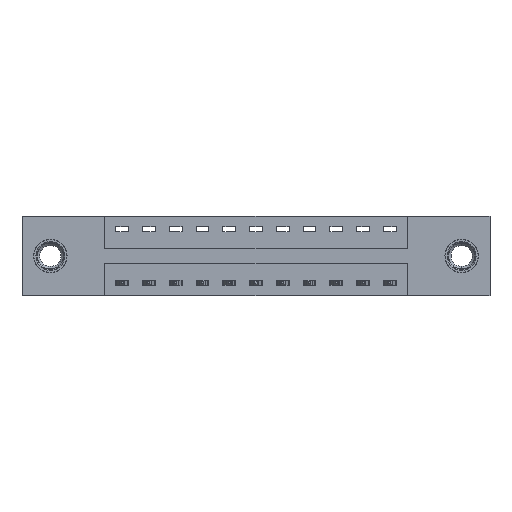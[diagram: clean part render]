
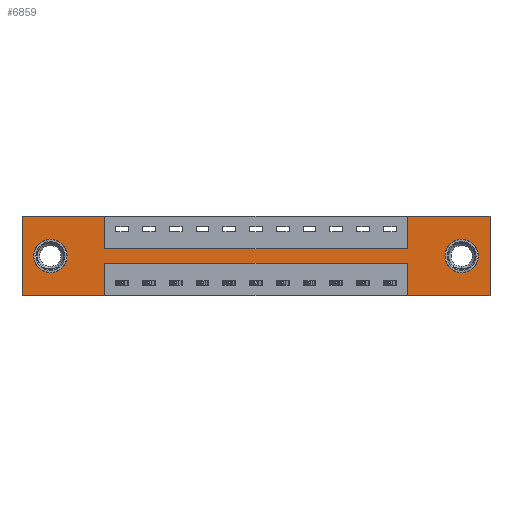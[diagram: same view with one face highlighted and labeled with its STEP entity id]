
A CAD part, front view. The second image highlights one B-rep face of the part: STEP entity #6859.
In plain terms, the highlighted planar face has unit normal (0, -1, 0).
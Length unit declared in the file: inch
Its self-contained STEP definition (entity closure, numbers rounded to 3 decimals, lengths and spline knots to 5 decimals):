
#109 = VERTEX_POINT ( 'NONE', #2069 ) ;
#162 = VERTEX_POINT ( 'NONE', #5123 ) ;
#343 = ORIENTED_EDGE ( 'NONE', *, *, #11135, .F. ) ;
#410 = CARTESIAN_POINT ( 'NONE',  ( 1.7975, 0., -0.15 ) ) ;
#486 = CARTESIAN_POINT ( 'NONE',  ( 1.7975, 0., -0.22 ) ) ;
#488 = EDGE_CURVE ( 'NONE', #7572, #2030, #11193, .T. ) ;
#491 = ORIENTED_EDGE ( 'NONE', *, *, #5879, .F. ) ;
#593 = VERTEX_POINT ( 'NONE', #3154 ) ;
#762 = CARTESIAN_POINT ( 'NONE',  ( 0.1325, 0., -0.185 ) ) ;
#849 = DIRECTION ( 'NONE',  ( 0., 0., 1. ) ) ;
#923 = CARTESIAN_POINT ( 'NONE',  ( 0., 0., 0. ) ) ;
#945 = LINE ( 'NONE', #8394, #10133 ) ;
#1381 = CARTESIAN_POINT ( 'NONE',  ( 0., 0., -0.37 ) ) ;
#1407 = CARTESIAN_POINT ( 'NONE',  ( 2.185, 0., 0. ) ) ;
#1415 = VECTOR ( 'NONE', #11627, 39.37008 ) ;
#1430 = ORIENTED_EDGE ( 'NONE', *, *, #6796, .F. ) ;
#1726 = LINE ( 'NONE', #923, #4914 ) ;
#1750 = DIRECTION ( 'NONE',  ( 0., -1., 0. ) ) ;
#1914 = VECTOR ( 'NONE', #849, 39.37008 ) ;
#1993 = FACE_OUTER_BOUND ( 'NONE', #2025, .T. ) ;
#2002 = LINE ( 'NONE', #5742, #10921 ) ;
#2025 = EDGE_LOOP ( 'NONE', ( #8663, #9573, #8241, #4562, #7363, #1430, #6151, #2543, #343, #491, #8839, #10587 ) ) ;
#2030 = VERTEX_POINT ( 'NONE', #11125 ) ;
#2040 = CARTESIAN_POINT ( 'NONE',  ( 2.0525, 0., -0.185 ) ) ;
#2069 = CARTESIAN_POINT ( 'NONE',  ( 0.3875, 0., 0. ) ) ;
#2076 = LINE ( 'NONE', #5697, #12197 ) ;
#2270 = DIRECTION ( 'NONE',  ( 0., 0., -1. ) ) ;
#2543 = ORIENTED_EDGE ( 'NONE', *, *, #9388, .F. ) ;
#2697 = DIRECTION ( 'NONE',  ( 0., 0., 1. ) ) ;
#2711 = DIRECTION ( 'NONE',  ( 0., 0., 1. ) ) ;
#2770 = CARTESIAN_POINT ( 'NONE',  ( 2.0525, 0., -0.107 ) ) ;
#2814 = ORIENTED_EDGE ( 'NONE', *, *, #6087, .T. ) ;
#2875 = VERTEX_POINT ( 'NONE', #1407 ) ;
#2902 = AXIS2_PLACEMENT_3D ( 'NONE', #3178, #3237, #8682 ) ;
#3089 = EDGE_CURVE ( 'NONE', #2030, #11890, #2076, .T. ) ;
#3128 = CARTESIAN_POINT ( 'NONE',  ( 2.0525, 0., -0.185 ) ) ;
#3154 = CARTESIAN_POINT ( 'NONE',  ( 1.7975, 0., 0. ) ) ;
#3178 = CARTESIAN_POINT ( 'NONE',  ( 0.1325, 0., -0.185 ) ) ;
#3237 = DIRECTION ( 'NONE',  ( 0., 1., 0. ) ) ;
#3247 = VERTEX_POINT ( 'NONE', #5873 ) ;
#3268 = VERTEX_POINT ( 'NONE', #410 ) ;
#3356 = VERTEX_POINT ( 'NONE', #9213 ) ;
#3519 = VECTOR ( 'NONE', #10197, 39.37008 ) ;
#3606 = CARTESIAN_POINT ( 'NONE',  ( 1.7975, 0., -0.37 ) ) ;
#3637 = FACE_BOUND ( 'NONE', #6050, .T. ) ;
#3666 = CARTESIAN_POINT ( 'NONE',  ( 1.7975, 0., 0. ) ) ;
#3793 = EDGE_LOOP ( 'NONE', ( #6740, #9868 ) ) ;
#3900 = DIRECTION ( 'NONE',  ( 0., 0., -1. ) ) ;
#3926 = DIRECTION ( 'NONE',  ( 0., 1., 0. ) ) ;
#3934 = VECTOR ( 'NONE', #11896, 39.37008 ) ;
#4210 = EDGE_CURVE ( 'NONE', #3247, #7572, #10282, .T. ) ;
#4308 = ORIENTED_EDGE ( 'NONE', *, *, #9092, .T. ) ;
#4513 = LINE ( 'NONE', #6518, #3519 ) ;
#4562 = ORIENTED_EDGE ( 'NONE', *, *, #5497, .F. ) ;
#4636 = PLANE ( 'NONE',  #8468 ) ;
#4914 = VECTOR ( 'NONE', #2697, 39.37008 ) ;
#5080 = CARTESIAN_POINT ( 'NONE',  ( 0.3875, 0., 0. ) ) ;
#5123 = CARTESIAN_POINT ( 'NONE',  ( 0.3875, 0., -0.15 ) ) ;
#5287 = AXIS2_PLACEMENT_3D ( 'NONE', #762, #6454, #2711 ) ;
#5389 = VECTOR ( 'NONE', #12076, 39.37008 ) ;
#5497 = EDGE_CURVE ( 'NONE', #6652, #3247, #945, .T. ) ;
#5555 = DIRECTION ( 'NONE',  ( -1., 0., 0. ) ) ;
#5577 = LINE ( 'NONE', #5764, #11763 ) ;
#5638 = DIRECTION ( 'NONE',  ( 1., 0., 0. ) ) ;
#5697 = CARTESIAN_POINT ( 'NONE',  ( 0.3875, 0., -0.37 ) ) ;
#5719 = VECTOR ( 'NONE', #2270, 39.37008 ) ;
#5742 = CARTESIAN_POINT ( 'NONE',  ( 2.185, 0., 0. ) ) ;
#5764 = CARTESIAN_POINT ( 'NONE',  ( 0., 0., 0. ) ) ;
#5814 = VERTEX_POINT ( 'NONE', #12082 ) ;
#5824 = LINE ( 'NONE', #3666, #1914 ) ;
#5873 = CARTESIAN_POINT ( 'NONE',  ( 1.7975, 0., -0.37 ) ) ;
#5879 = EDGE_CURVE ( 'NONE', #5814, #109, #5577, .T. ) ;
#5960 = EDGE_CURVE ( 'NONE', #3268, #593, #5824, .T. ) ;
#6050 = EDGE_LOOP ( 'NONE', ( #2814, #4308 ) ) ;
#6086 = VERTEX_POINT ( 'NONE', #11643 ) ;
#6087 = EDGE_CURVE ( 'NONE', #6086, #7773, #8229, .T. ) ;
#6151 = ORIENTED_EDGE ( 'NONE', *, *, #5960, .F. ) ;
#6187 = VECTOR ( 'NONE', #5555, 39.37008 ) ;
#6408 = CARTESIAN_POINT ( 'NONE',  ( 0., 0., -0.37 ) ) ;
#6454 = DIRECTION ( 'NONE',  ( 0., 1., 0. ) ) ;
#6518 = CARTESIAN_POINT ( 'NONE',  ( 0., 0., 0. ) ) ;
#6652 = VERTEX_POINT ( 'NONE', #7090 ) ;
#6680 = DIRECTION ( 'NONE',  ( 0., 0., -1. ) ) ;
#6740 = ORIENTED_EDGE ( 'NONE', *, *, #9245, .T. ) ;
#6756 = DIRECTION ( 'NONE',  ( 0., 1., 0. ) ) ;
#6762 = CARTESIAN_POINT ( 'NONE',  ( 0.3875, 0., -0.37 ) ) ;
#6796 = EDGE_CURVE ( 'NONE', #593, #2875, #4513, .T. ) ;
#6859 = ADVANCED_FACE ( 'NONE', ( #10441, #3637, #1993 ), #4636, .T. ) ;
#7090 = CARTESIAN_POINT ( 'NONE',  ( 2.185, 0., -0.37 ) ) ;
#7333 = DIRECTION ( 'NONE',  ( -1., 0., 0. ) ) ;
#7363 = ORIENTED_EDGE ( 'NONE', *, *, #10090, .F. ) ;
#7453 = DIRECTION ( 'NONE',  ( 0., 0., -1. ) ) ;
#7572 = VERTEX_POINT ( 'NONE', #486 ) ;
#7697 = DIRECTION ( 'NONE',  ( 0., 0., -1. ) ) ;
#7773 = VERTEX_POINT ( 'NONE', #11632 ) ;
#7898 = AXIS2_PLACEMENT_3D ( 'NONE', #2040, #6756, #7697 ) ;
#8229 = CIRCLE ( 'NONE', #2902, 0.078 ) ;
#8241 = ORIENTED_EDGE ( 'NONE', *, *, #4210, .F. ) ;
#8267 = CIRCLE ( 'NONE', #5287, 0.078 ) ;
#8394 = CARTESIAN_POINT ( 'NONE',  ( 0., 0., -0.37 ) ) ;
#8468 = AXIS2_PLACEMENT_3D ( 'NONE', #6408, #1750, #7453 ) ;
#8557 = VERTEX_POINT ( 'NONE', #2770 ) ;
#8663 = ORIENTED_EDGE ( 'NONE', *, *, #3089, .F. ) ;
#8682 = DIRECTION ( 'NONE',  ( 0., 0., 1. ) ) ;
#8786 = LINE ( 'NONE', #1381, #1415 ) ;
#8839 = ORIENTED_EDGE ( 'NONE', *, *, #10799, .F. ) ;
#9092 = EDGE_CURVE ( 'NONE', #7773, #6086, #8267, .T. ) ;
#9213 = CARTESIAN_POINT ( 'NONE',  ( 0., 0., -0.37 ) ) ;
#9245 = EDGE_CURVE ( 'NONE', #8557, #9983, #10474, .T. ) ;
#9388 = EDGE_CURVE ( 'NONE', #162, #3268, #11095, .T. ) ;
#9494 = AXIS2_PLACEMENT_3D ( 'NONE', #3128, #3926, #6680 ) ;
#9573 = ORIENTED_EDGE ( 'NONE', *, *, #488, .F. ) ;
#9868 = ORIENTED_EDGE ( 'NONE', *, *, #11057, .T. ) ;
#9983 = VERTEX_POINT ( 'NONE', #12121 ) ;
#10076 = CIRCLE ( 'NONE', #9494, 0.078 ) ;
#10090 = EDGE_CURVE ( 'NONE', #2875, #6652, #2002, .T. ) ;
#10133 = VECTOR ( 'NONE', #7333, 39.37008 ) ;
#10197 = DIRECTION ( 'NONE',  ( 1., 0., 0. ) ) ;
#10263 = CARTESIAN_POINT ( 'NONE',  ( 0.3875, 0., -0.22 ) ) ;
#10281 = DIRECTION ( 'NONE',  ( 0., 0., -1. ) ) ;
#10282 = LINE ( 'NONE', #3606, #3934 ) ;
#10441 = FACE_BOUND ( 'NONE', #3793, .T. ) ;
#10474 = CIRCLE ( 'NONE', #7898, 0.078 ) ;
#10587 = ORIENTED_EDGE ( 'NONE', *, *, #11397, .F. ) ;
#10799 = EDGE_CURVE ( 'NONE', #3356, #5814, #1726, .T. ) ;
#10912 = LINE ( 'NONE', #5080, #5719 ) ;
#10921 = VECTOR ( 'NONE', #3900, 39.37008 ) ;
#11057 = EDGE_CURVE ( 'NONE', #9983, #8557, #10076, .T. ) ;
#11095 = LINE ( 'NONE', #12018, #5389 ) ;
#11125 = CARTESIAN_POINT ( 'NONE',  ( 0.3875, 0., -0.22 ) ) ;
#11135 = EDGE_CURVE ( 'NONE', #109, #162, #10912, .T. ) ;
#11193 = LINE ( 'NONE', #10263, #6187 ) ;
#11397 = EDGE_CURVE ( 'NONE', #11890, #3356, #8786, .T. ) ;
#11627 = DIRECTION ( 'NONE',  ( -1., 0., 0. ) ) ;
#11632 = CARTESIAN_POINT ( 'NONE',  ( 0.1325, 0., -0.263 ) ) ;
#11643 = CARTESIAN_POINT ( 'NONE',  ( 0.1325, 0., -0.107 ) ) ;
#11763 = VECTOR ( 'NONE', #5638, 39.37008 ) ;
#11890 = VERTEX_POINT ( 'NONE', #6762 ) ;
#11896 = DIRECTION ( 'NONE',  ( 0., 0., 1. ) ) ;
#12018 = CARTESIAN_POINT ( 'NONE',  ( 0.3875, 0., -0.15 ) ) ;
#12076 = DIRECTION ( 'NONE',  ( 1., 0., 0. ) ) ;
#12082 = CARTESIAN_POINT ( 'NONE',  ( 0., 0., 0. ) ) ;
#12121 = CARTESIAN_POINT ( 'NONE',  ( 2.0525, 0., -0.263 ) ) ;
#12197 = VECTOR ( 'NONE', #10281, 39.37008 ) ;
